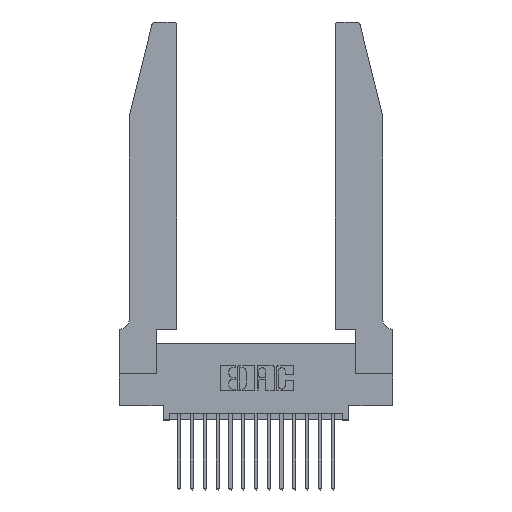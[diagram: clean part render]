
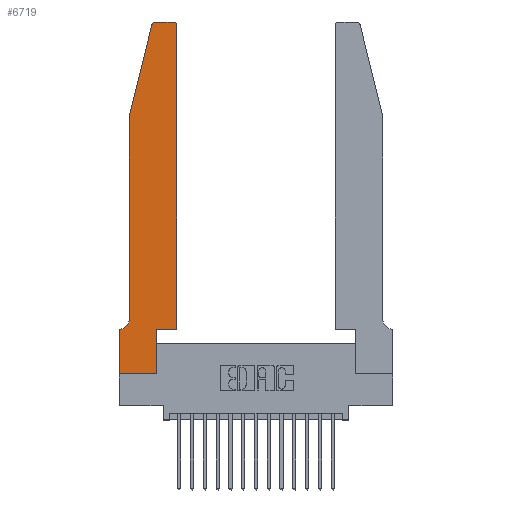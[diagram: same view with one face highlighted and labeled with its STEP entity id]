
A CAD part, top view. The second image highlights one B-rep face of the part: STEP entity #6719.
In plain terms, the highlighted planar face has unit normal (0, 0, 1).
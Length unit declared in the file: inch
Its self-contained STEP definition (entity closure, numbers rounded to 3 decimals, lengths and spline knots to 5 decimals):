
#175 = EDGE_CURVE ( 'NONE', #8891, #5475, #18656, .T. ) ;
#237 = EDGE_CURVE ( 'NONE', #12769, #8891, #10532, .T. ) ;
#399 = VERTEX_POINT ( 'NONE', #8855 ) ;
#445 = CARTESIAN_POINT ( 'NONE',  ( 0.4505, 2.72, 0.37 ) ) ;
#794 = CARTESIAN_POINT ( 'NONE',  ( 0.0755, 2., 0.37 ) ) ;
#1002 = CARTESIAN_POINT ( 'NONE',  ( 0.0055, 0.42, 0.37 ) ) ;
#1176 = DIRECTION ( 'NONE',  ( -1., 0., 0. ) ) ;
#1223 = DIRECTION ( 'NONE',  ( 0., 0., -1. ) ) ;
#1255 = EDGE_CURVE ( 'NONE', #5475, #18128, #3870, .T. ) ;
#1504 = EDGE_CURVE ( 'NONE', #9872, #12769, #4103, .T. ) ;
#1520 = VECTOR ( 'NONE', #13222, 39.37008 ) ;
#1722 = EDGE_LOOP ( 'NONE', ( #8297, #14869, #13789, #11902, #10665, #5036, #14266, #1806, #11154, #6989, #17379, #6822 ) ) ;
#1739 = DIRECTION ( 'NONE',  ( 0., -1., 0. ) ) ;
#1788 = VERTEX_POINT ( 'NONE', #8829 ) ;
#1806 = ORIENTED_EDGE ( 'NONE', *, *, #10555, .T. ) ;
#1816 = CARTESIAN_POINT ( 'NONE',  ( 0.2605, 2.75, 0.37 ) ) ;
#1885 = CARTESIAN_POINT ( 'NONE',  ( 0., 0.35, 0.37 ) ) ;
#1973 = DIRECTION ( 'NONE',  ( 0., 0., 1. ) ) ;
#1999 = CARTESIAN_POINT ( 'NONE',  ( 0.284, 2.72, 0.37 ) ) ;
#2035 = LINE ( 'NONE', #10808, #6239 ) ;
#2179 = DIRECTION ( 'NONE',  ( 1., 0., 0. ) ) ;
#2192 = LINE ( 'NONE', #1816, #17171 ) ;
#2760 = CARTESIAN_POINT ( 'NONE',  ( 0.2865, 0.35, 0.37 ) ) ;
#2926 = CARTESIAN_POINT ( 'NONE',  ( 0.25487, 2.72718, 0.37 ) ) ;
#3267 = VECTOR ( 'NONE', #18196, 39.37008 ) ;
#3513 = DIRECTION ( 'NONE',  ( 1., 0., 0. ) ) ;
#3870 = CIRCLE ( 'NONE', #14182, 0.07 ) ;
#4103 = CIRCLE ( 'NONE', #8239, 0.03 ) ;
#5036 = ORIENTED_EDGE ( 'NONE', *, *, #7866, .T. ) ;
#5293 = VERTEX_POINT ( 'NONE', #12208 ) ;
#5418 = VECTOR ( 'NONE', #8257, 39.37008 ) ;
#5475 = VERTEX_POINT ( 'NONE', #8372 ) ;
#5751 = VECTOR ( 'NONE', #14655, 39.37008 ) ;
#6239 = VECTOR ( 'NONE', #12184, 39.37008 ) ;
#6381 = DIRECTION ( 'NONE',  ( 0., 0., 1. ) ) ;
#6545 = AXIS2_PLACEMENT_3D ( 'NONE', #14876, #6381, #16215 ) ;
#6590 = PLANE ( 'NONE',  #18498 ) ;
#6715 = CARTESIAN_POINT ( 'NONE',  ( 0.4505, 0.35, 0.37 ) ) ;
#6719 = ADVANCED_FACE ( 'NONE', ( #8681 ), #6590, .T. ) ;
#6822 = ORIENTED_EDGE ( 'NONE', *, *, #17750, .T. ) ;
#6989 = ORIENTED_EDGE ( 'NONE', *, *, #17916, .T. ) ;
#7086 = VECTOR ( 'NONE', #1739, 39.37008 ) ;
#7158 = DIRECTION ( 'NONE',  ( 0., 1., 0. ) ) ;
#7866 = EDGE_CURVE ( 'NONE', #18128, #14598, #2035, .T. ) ;
#8239 = AXIS2_PLACEMENT_3D ( 'NONE', #1999, #1973, #2179 ) ;
#8257 = DIRECTION ( 'NONE',  ( 1., 0., 0. ) ) ;
#8297 = ORIENTED_EDGE ( 'NONE', *, *, #17852, .T. ) ;
#8372 = CARTESIAN_POINT ( 'NONE',  ( 0.0755, 0.42, 0.37 ) ) ;
#8681 = FACE_OUTER_BOUND ( 'NONE', #1722, .T. ) ;
#8751 = DIRECTION ( 'NONE',  ( -0.239, -0.971, 0. ) ) ;
#8829 = CARTESIAN_POINT ( 'NONE',  ( 0.2865, 0.35, 0.37 ) ) ;
#8855 = CARTESIAN_POINT ( 'NONE',  ( 0.4205, 2.75, 0.37 ) ) ;
#8891 = VERTEX_POINT ( 'NONE', #14433 ) ;
#9490 = EDGE_CURVE ( 'NONE', #13845, #1788, #9781, .T. ) ;
#9514 = EDGE_CURVE ( 'NONE', #14598, #5293, #12999, .T. ) ;
#9663 = VECTOR ( 'NONE', #8751, 39.37008 ) ;
#9781 = LINE ( 'NONE', #2760, #1520 ) ;
#9872 = VERTEX_POINT ( 'NONE', #11316 ) ;
#10012 = CARTESIAN_POINT ( 'NONE',  ( 0., 0., 0.37 ) ) ;
#10460 = VERTEX_POINT ( 'NONE', #445 ) ;
#10532 = LINE ( 'NONE', #14792, #9663 ) ;
#10555 = EDGE_CURVE ( 'NONE', #5293, #13845, #14875, .T. ) ;
#10665 = ORIENTED_EDGE ( 'NONE', *, *, #1255, .T. ) ;
#10808 = CARTESIAN_POINT ( 'NONE',  ( 0.0755, 0.35, 0.37 ) ) ;
#11154 = ORIENTED_EDGE ( 'NONE', *, *, #9490, .T. ) ;
#11316 = CARTESIAN_POINT ( 'NONE',  ( 0.284, 2.75, 0.37 ) ) ;
#11902 = ORIENTED_EDGE ( 'NONE', *, *, #175, .T. ) ;
#12184 = DIRECTION ( 'NONE',  ( -1., 0., 0. ) ) ;
#12208 = CARTESIAN_POINT ( 'NONE',  ( 0., 0., 0.37 ) ) ;
#12399 = DIRECTION ( 'NONE',  ( 0., 0., 1. ) ) ;
#12769 = VERTEX_POINT ( 'NONE', #2926 ) ;
#12999 = LINE ( 'NONE', #17395, #5751 ) ;
#13154 = VECTOR ( 'NONE', #7158, 39.37008 ) ;
#13222 = DIRECTION ( 'NONE',  ( 0., 1., 0. ) ) ;
#13789 = ORIENTED_EDGE ( 'NONE', *, *, #237, .T. ) ;
#13845 = VERTEX_POINT ( 'NONE', #18650 ) ;
#14003 = LINE ( 'NONE', #16916, #13154 ) ;
#14182 = AXIS2_PLACEMENT_3D ( 'NONE', #1002, #1223, #1176 ) ;
#14266 = ORIENTED_EDGE ( 'NONE', *, *, #9514, .T. ) ;
#14400 = LINE ( 'NONE', #6715, #5418 ) ;
#14433 = CARTESIAN_POINT ( 'NONE',  ( 0.0755, 2., 0.37 ) ) ;
#14598 = VERTEX_POINT ( 'NONE', #18104 ) ;
#14655 = DIRECTION ( 'NONE',  ( 0., -1., 0. ) ) ;
#14792 = CARTESIAN_POINT ( 'NONE',  ( 0.0755, 2., 0.37 ) ) ;
#14869 = ORIENTED_EDGE ( 'NONE', *, *, #1504, .T. ) ;
#14875 = LINE ( 'NONE', #10012, #3267 ) ;
#14876 = CARTESIAN_POINT ( 'NONE',  ( 0.4205, 2.72, 0.37 ) ) ;
#15039 = DIRECTION ( 'NONE',  ( -1., 0., 0. ) ) ;
#16072 = CIRCLE ( 'NONE', #6545, 0.03 ) ;
#16215 = DIRECTION ( 'NONE',  ( 1., 0., 0. ) ) ;
#16332 = VERTEX_POINT ( 'NONE', #18382 ) ;
#16916 = CARTESIAN_POINT ( 'NONE',  ( 0.4505, 0.35, 0.37 ) ) ;
#16987 = EDGE_CURVE ( 'NONE', #16332, #10460, #14003, .T. ) ;
#16999 = CARTESIAN_POINT ( 'NONE',  ( 0.0055, 0.35, 0.37 ) ) ;
#17171 = VECTOR ( 'NONE', #15039, 39.37008 ) ;
#17379 = ORIENTED_EDGE ( 'NONE', *, *, #16987, .T. ) ;
#17395 = CARTESIAN_POINT ( 'NONE',  ( 0., 0., 0.37 ) ) ;
#17750 = EDGE_CURVE ( 'NONE', #10460, #399, #16072, .T. ) ;
#17852 = EDGE_CURVE ( 'NONE', #399, #9872, #2192, .T. ) ;
#17916 = EDGE_CURVE ( 'NONE', #1788, #16332, #14400, .T. ) ;
#18104 = CARTESIAN_POINT ( 'NONE',  ( 0., 0.35, 0.37 ) ) ;
#18128 = VERTEX_POINT ( 'NONE', #16999 ) ;
#18196 = DIRECTION ( 'NONE',  ( 1., 0., 0. ) ) ;
#18382 = CARTESIAN_POINT ( 'NONE',  ( 0.4505, 0.35, 0.37 ) ) ;
#18498 = AXIS2_PLACEMENT_3D ( 'NONE', #1885, #12399, #3513 ) ;
#18650 = CARTESIAN_POINT ( 'NONE',  ( 0.2865, 0., 0.37 ) ) ;
#18656 = LINE ( 'NONE', #794, #7086 ) ;
